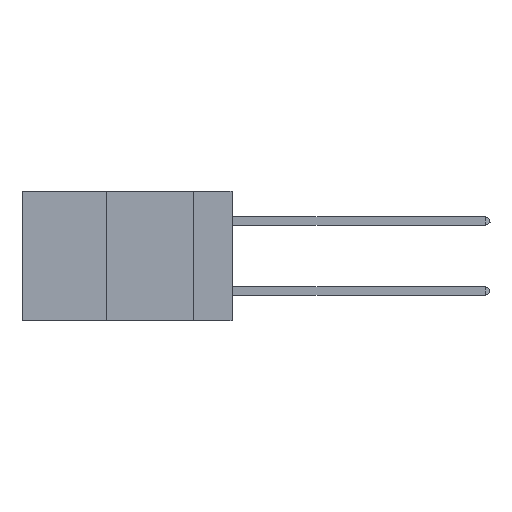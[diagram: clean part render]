
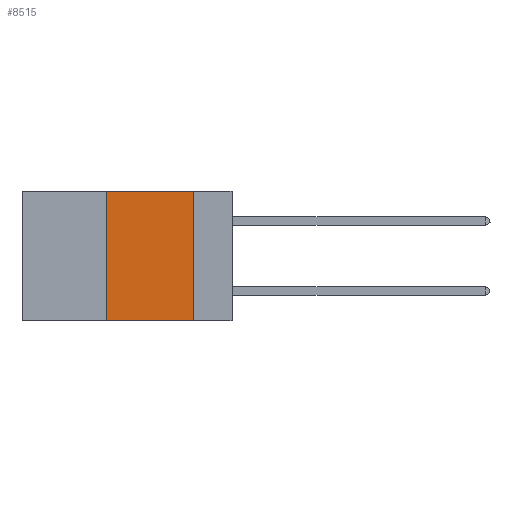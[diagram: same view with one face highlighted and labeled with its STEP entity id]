
A CAD part, left-side view. The second image highlights one B-rep face of the part: STEP entity #8515.
In plain terms, the highlighted planar face has unit normal (-1, 0, 0).
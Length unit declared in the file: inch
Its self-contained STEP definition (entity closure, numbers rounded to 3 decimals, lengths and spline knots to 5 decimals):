
#6 = DIRECTION ( 'NONE',  ( 0., -1., 0. ) ) ;
#886 = AXIS2_PLACEMENT_3D ( 'NONE', #18083, #2277, #33785 ) ;
#930 = LINE ( 'NONE', #25815, #23355 ) ;
#2277 = DIRECTION ( 'NONE',  ( 1., 0., 0. ) ) ;
#2529 = CARTESIAN_POINT ( 'NONE',  ( 0., 0.36, -0.37 ) ) ;
#2730 = ORIENTED_EDGE ( 'NONE', *, *, #12139, .F. ) ;
#3012 = VECTOR ( 'NONE', #8133, 39.37008 ) ;
#4006 = EDGE_CURVE ( 'NONE', #20271, #18515, #4373, .T. ) ;
#4248 = CARTESIAN_POINT ( 'NONE',  ( 0., 0.36, 0. ) ) ;
#4373 = LINE ( 'NONE', #33513, #10223 ) ;
#6711 = EDGE_CURVE ( 'NONE', #29891, #11718, #930, .T. ) ;
#8058 = VECTOR ( 'NONE', #26461, 39.37008 ) ;
#8133 = DIRECTION ( 'NONE',  ( 0., 0., -1. ) ) ;
#8515 = ADVANCED_FACE ( 'NONE', ( #17844 ), #11833, .F. ) ;
#10223 = VECTOR ( 'NONE', #17563, 39.37008 ) ;
#11416 = ORIENTED_EDGE ( 'NONE', *, *, #6711, .F. ) ;
#11718 = VERTEX_POINT ( 'NONE', #19287 ) ;
#11833 = PLANE ( 'NONE',  #886 ) ;
#12139 = EDGE_CURVE ( 'NONE', #11718, #18515, #32161, .T. ) ;
#14508 = CARTESIAN_POINT ( 'NONE',  ( 0., 0.11, -0.37 ) ) ;
#16588 = ORIENTED_EDGE ( 'NONE', *, *, #4006, .T. ) ;
#17563 = DIRECTION ( 'NONE',  ( 0., -1., 0. ) ) ;
#17844 = FACE_OUTER_BOUND ( 'NONE', #26659, .T. ) ;
#18083 = CARTESIAN_POINT ( 'NONE',  ( 0., 0.6, 0. ) ) ;
#18515 = VERTEX_POINT ( 'NONE', #14508 ) ;
#19287 = CARTESIAN_POINT ( 'NONE',  ( 0., 0.11, 0. ) ) ;
#20271 = VERTEX_POINT ( 'NONE', #2529 ) ;
#23355 = VECTOR ( 'NONE', #6, 39.37008 ) ;
#23986 = CARTESIAN_POINT ( 'NONE',  ( 0., 0.36, 0. ) ) ;
#24243 = LINE ( 'NONE', #23986, #8058 ) ;
#25815 = CARTESIAN_POINT ( 'NONE',  ( 0., 0.6, 0. ) ) ;
#26390 = ORIENTED_EDGE ( 'NONE', *, *, #26495, .F. ) ;
#26461 = DIRECTION ( 'NONE',  ( 0., 0., 1. ) ) ;
#26495 = EDGE_CURVE ( 'NONE', #20271, #29891, #24243, .T. ) ;
#26659 = EDGE_LOOP ( 'NONE', ( #2730, #11416, #26390, #16588 ) ) ;
#27184 = CARTESIAN_POINT ( 'NONE',  ( 0., 0.11, 0. ) ) ;
#29891 = VERTEX_POINT ( 'NONE', #4248 ) ;
#32161 = LINE ( 'NONE', #27184, #3012 ) ;
#33513 = CARTESIAN_POINT ( 'NONE',  ( 0., 0.6, -0.37 ) ) ;
#33785 = DIRECTION ( 'NONE',  ( 0., 0., -1. ) ) ;
